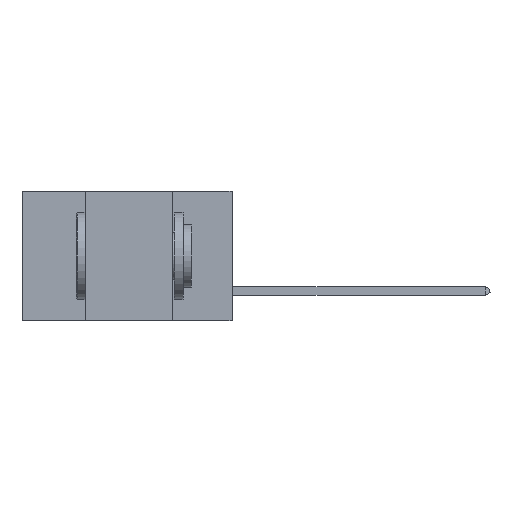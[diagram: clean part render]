
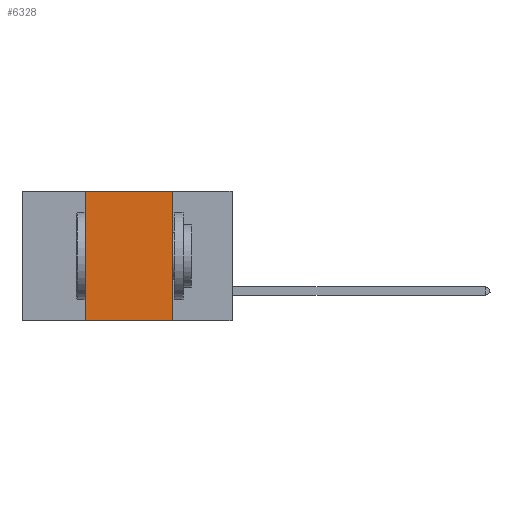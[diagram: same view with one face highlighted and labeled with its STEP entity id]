
A CAD part, left-side view. The second image highlights one B-rep face of the part: STEP entity #6328.
In plain terms, the highlighted planar face has unit normal (-1, 0, 0).
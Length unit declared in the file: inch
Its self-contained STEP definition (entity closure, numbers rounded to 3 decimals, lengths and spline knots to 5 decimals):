
#526 = VECTOR ( 'NONE', #17189, 39.37008 ) ;
#764 = CARTESIAN_POINT ( 'NONE',  ( 0., 0.42, 0. ) ) ;
#930 = VERTEX_POINT ( 'NONE', #25913 ) ;
#1670 = CARTESIAN_POINT ( 'NONE',  ( 0., 0.6, -0.37 ) ) ;
#1922 = ORIENTED_EDGE ( 'NONE', *, *, #8391, .F. ) ;
#3004 = LINE ( 'NONE', #20112, #20224 ) ;
#3240 = EDGE_CURVE ( 'NONE', #24196, #7831, #7524, .T. ) ;
#3454 = CARTESIAN_POINT ( 'NONE',  ( 0., 0.17, 0. ) ) ;
#5314 = ORIENTED_EDGE ( 'NONE', *, *, #23411, .T. ) ;
#5631 = PLANE ( 'NONE',  #24993 ) ;
#5759 = FACE_OUTER_BOUND ( 'NONE', #24970, .T. ) ;
#6103 = DIRECTION ( 'NONE',  ( 0., -1., 0. ) ) ;
#6328 = ADVANCED_FACE ( 'NONE', ( #5759 ), #5631, .F. ) ;
#6591 = EDGE_CURVE ( 'NONE', #7831, #17231, #15733, .T. ) ;
#7524 = LINE ( 'NONE', #11300, #26324 ) ;
#7727 = DIRECTION ( 'NONE',  ( 1., 0., 0. ) ) ;
#7831 = VERTEX_POINT ( 'NONE', #764 ) ;
#8391 = EDGE_CURVE ( 'NONE', #17231, #930, #3004, .T. ) ;
#9138 = VECTOR ( 'NONE', #6103, 39.37008 ) ;
#11071 = CARTESIAN_POINT ( 'NONE',  ( 0., 0.42, -0.37 ) ) ;
#11300 = CARTESIAN_POINT ( 'NONE',  ( 0., 0.42, 0. ) ) ;
#12106 = DIRECTION ( 'NONE',  ( 0., 0., -1. ) ) ;
#13661 = ORIENTED_EDGE ( 'NONE', *, *, #6591, .F. ) ;
#15733 = LINE ( 'NONE', #18510, #526 ) ;
#17189 = DIRECTION ( 'NONE',  ( 0., -1., 0. ) ) ;
#17231 = VERTEX_POINT ( 'NONE', #3454 ) ;
#18510 = CARTESIAN_POINT ( 'NONE',  ( 0., 0.6, 0. ) ) ;
#20112 = CARTESIAN_POINT ( 'NONE',  ( 0., 0.17, 0. ) ) ;
#20114 = CARTESIAN_POINT ( 'NONE',  ( 0., 0.6, 0. ) ) ;
#20224 = VECTOR ( 'NONE', #12106, 39.37008 ) ;
#22760 = LINE ( 'NONE', #1670, #9138 ) ;
#23411 = EDGE_CURVE ( 'NONE', #24196, #930, #22760, .T. ) ;
#24196 = VERTEX_POINT ( 'NONE', #11071 ) ;
#24970 = EDGE_LOOP ( 'NONE', ( #1922, #13661, #25647, #5314 ) ) ;
#24993 = AXIS2_PLACEMENT_3D ( 'NONE', #20114, #7727, #26386 ) ;
#25647 = ORIENTED_EDGE ( 'NONE', *, *, #3240, .F. ) ;
#25913 = CARTESIAN_POINT ( 'NONE',  ( 0., 0.17, -0.37 ) ) ;
#26001 = DIRECTION ( 'NONE',  ( 0., 0., 1. ) ) ;
#26324 = VECTOR ( 'NONE', #26001, 39.37008 ) ;
#26386 = DIRECTION ( 'NONE',  ( 0., 0., -1. ) ) ;
